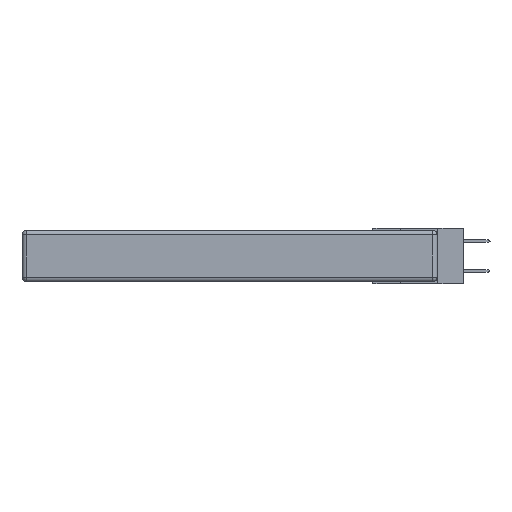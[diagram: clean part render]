
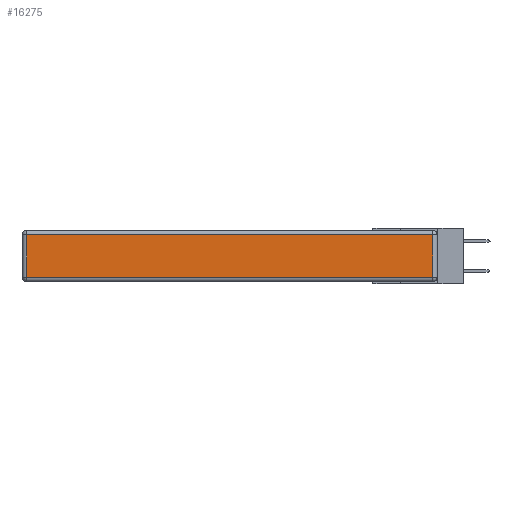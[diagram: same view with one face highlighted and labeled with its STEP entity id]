
A CAD part, left-side view. The second image highlights one B-rep face of the part: STEP entity #16275.
In plain terms, the highlighted planar face has unit normal (-1, 0, 0).
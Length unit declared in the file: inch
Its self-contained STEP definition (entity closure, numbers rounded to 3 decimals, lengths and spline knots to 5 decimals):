
#777 = EDGE_CURVE ( 'NONE', #3785, #18157, #4019, .T. ) ;
#1818 = DIRECTION ( 'NONE',  ( 0., 1., 0. ) ) ;
#1961 = VECTOR ( 'NONE', #9691, 39.37008 ) ;
#2955 = DIRECTION ( 'NONE',  ( 0., -1., 0. ) ) ;
#3482 = VERTEX_POINT ( 'NONE', #18269 ) ;
#3660 = EDGE_CURVE ( 'NONE', #18157, #3482, #11861, .T. ) ;
#3752 = CARTESIAN_POINT ( 'NONE',  ( 0., 2.72, -0.03 ) ) ;
#3785 = VERTEX_POINT ( 'NONE', #11640 ) ;
#4019 = LINE ( 'NONE', #6556, #10511 ) ;
#4256 = EDGE_CURVE ( 'NONE', #3482, #16209, #7033, .T. ) ;
#4288 = DIRECTION ( 'NONE',  ( 0., 0., 1. ) ) ;
#4371 = CARTESIAN_POINT ( 'NONE',  ( 0., 0., -0.343 ) ) ;
#4911 = CARTESIAN_POINT ( 'NONE',  ( 0., 0.03, -0.313 ) ) ;
#6556 = CARTESIAN_POINT ( 'NONE',  ( 0., 2.75, -0.03 ) ) ;
#6778 = LINE ( 'NONE', #8329, #14492 ) ;
#7033 = LINE ( 'NONE', #12192, #18393 ) ;
#7056 = ORIENTED_EDGE ( 'NONE', *, *, #3660, .T. ) ;
#8329 = CARTESIAN_POINT ( 'NONE',  ( 0., 0.03, -0.343 ) ) ;
#8993 = DIRECTION ( 'NONE',  ( -1., 0., 0. ) ) ;
#9691 = DIRECTION ( 'NONE',  ( 0., 0., -1. ) ) ;
#9808 = ORIENTED_EDGE ( 'NONE', *, *, #777, .T. ) ;
#10250 = PLANE ( 'NONE',  #14368 ) ;
#10511 = VECTOR ( 'NONE', #1818, 39.37008 ) ;
#11640 = CARTESIAN_POINT ( 'NONE',  ( 0., 0.03, -0.03 ) ) ;
#11861 = LINE ( 'NONE', #14294, #1961 ) ;
#12192 = CARTESIAN_POINT ( 'NONE',  ( 0., 0., -0.313 ) ) ;
#14294 = CARTESIAN_POINT ( 'NONE',  ( 0., 2.72, -0.343 ) ) ;
#14368 = AXIS2_PLACEMENT_3D ( 'NONE', #4371, #8993, #4288 ) ;
#14492 = VECTOR ( 'NONE', #15946, 39.37008 ) ;
#14840 = ORIENTED_EDGE ( 'NONE', *, *, #15567, .T. ) ;
#15567 = EDGE_CURVE ( 'NONE', #16209, #3785, #6778, .T. ) ;
#15696 = ORIENTED_EDGE ( 'NONE', *, *, #4256, .T. ) ;
#15946 = DIRECTION ( 'NONE',  ( 0., 0., 1. ) ) ;
#16209 = VERTEX_POINT ( 'NONE', #4911 ) ;
#16275 = ADVANCED_FACE ( 'NONE', ( #17629 ), #10250, .T. ) ;
#17629 = FACE_OUTER_BOUND ( 'NONE', #20012, .T. ) ;
#18157 = VERTEX_POINT ( 'NONE', #3752 ) ;
#18269 = CARTESIAN_POINT ( 'NONE',  ( 0., 2.72, -0.313 ) ) ;
#18393 = VECTOR ( 'NONE', #2955, 39.37008 ) ;
#20012 = EDGE_LOOP ( 'NONE', ( #15696, #14840, #9808, #7056 ) ) ;
